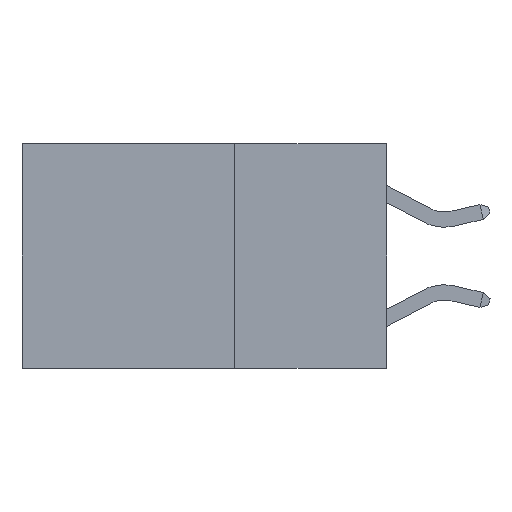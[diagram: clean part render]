
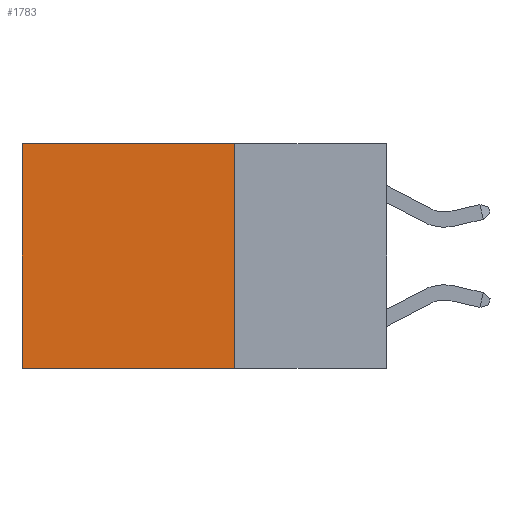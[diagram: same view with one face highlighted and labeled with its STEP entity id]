
A CAD part, left-side view. The second image highlights one B-rep face of the part: STEP entity #1783.
In plain terms, the highlighted planar face has unit normal (-1, 0, 0).
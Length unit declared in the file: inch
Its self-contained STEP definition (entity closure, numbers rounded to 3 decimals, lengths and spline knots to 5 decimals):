
#60 = ORIENTED_EDGE ( 'NONE', *, *, #17264, .T. ) ;
#1653 = EDGE_CURVE ( 'NONE', #19703, #4276, #16063, .T. ) ;
#1783 = ADVANCED_FACE ( 'NONE', ( #25073 ), #24254, .F. ) ;
#2023 = ORIENTED_EDGE ( 'NONE', *, *, #23006, .T. ) ;
#2615 = DIRECTION ( 'NONE',  ( 0., 0., -1. ) ) ;
#3171 = AXIS2_PLACEMENT_3D ( 'NONE', #10973, #13222, #28685 ) ;
#3690 = EDGE_CURVE ( 'NONE', #4276, #9024, #4072, .T. ) ;
#3721 = CARTESIAN_POINT ( 'NONE',  ( 0.2625, 0.25, 0. ) ) ;
#4072 = LINE ( 'NONE', #8043, #7970 ) ;
#4276 = VERTEX_POINT ( 'NONE', #25551 ) ;
#5268 = CARTESIAN_POINT ( 'NONE',  ( 0.2625, 0.25, 0. ) ) ;
#6698 = CARTESIAN_POINT ( 'NONE',  ( 0.2625, 0.6, 0. ) ) ;
#7944 = DIRECTION ( 'NONE',  ( 0., 1., 0. ) ) ;
#7970 = VECTOR ( 'NONE', #7944, 39.37008 ) ;
#8043 = CARTESIAN_POINT ( 'NONE',  ( 0.2625, 0.25, -0.37 ) ) ;
#9024 = VERTEX_POINT ( 'NONE', #25134 ) ;
#10145 = VECTOR ( 'NONE', #12757, 39.37008 ) ;
#10450 = EDGE_LOOP ( 'NONE', ( #60, #20946, #28257, #2023 ) ) ;
#10973 = CARTESIAN_POINT ( 'NONE',  ( 0.2625, 0.25, 0. ) ) ;
#12757 = DIRECTION ( 'NONE',  ( 0., 0., -1. ) ) ;
#13222 = DIRECTION ( 'NONE',  ( 1., 0., 0. ) ) ;
#14665 = LINE ( 'NONE', #5268, #19857 ) ;
#14816 = VECTOR ( 'NONE', #2615, 39.37008 ) ;
#16063 = LINE ( 'NONE', #3721, #10145 ) ;
#17264 = EDGE_CURVE ( 'NONE', #22190, #9024, #22082, .T. ) ;
#19703 = VERTEX_POINT ( 'NONE', #23741 ) ;
#19857 = VECTOR ( 'NONE', #23058, 39.37008 ) ;
#20946 = ORIENTED_EDGE ( 'NONE', *, *, #3690, .F. ) ;
#22082 = LINE ( 'NONE', #24853, #14816 ) ;
#22190 = VERTEX_POINT ( 'NONE', #6698 ) ;
#23006 = EDGE_CURVE ( 'NONE', #19703, #22190, #14665, .T. ) ;
#23058 = DIRECTION ( 'NONE',  ( 0., 1., 0. ) ) ;
#23741 = CARTESIAN_POINT ( 'NONE',  ( 0.2625, 0.25, 0. ) ) ;
#24254 = PLANE ( 'NONE',  #3171 ) ;
#24853 = CARTESIAN_POINT ( 'NONE',  ( 0.2625, 0.6, 0. ) ) ;
#25073 = FACE_OUTER_BOUND ( 'NONE', #10450, .T. ) ;
#25134 = CARTESIAN_POINT ( 'NONE',  ( 0.2625, 0.6, -0.37 ) ) ;
#25551 = CARTESIAN_POINT ( 'NONE',  ( 0.2625, 0.25, -0.37 ) ) ;
#28257 = ORIENTED_EDGE ( 'NONE', *, *, #1653, .F. ) ;
#28685 = DIRECTION ( 'NONE',  ( 0., 0., -1. ) ) ;
